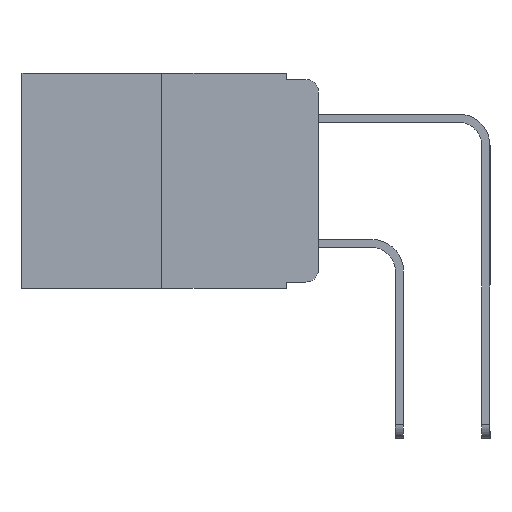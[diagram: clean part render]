
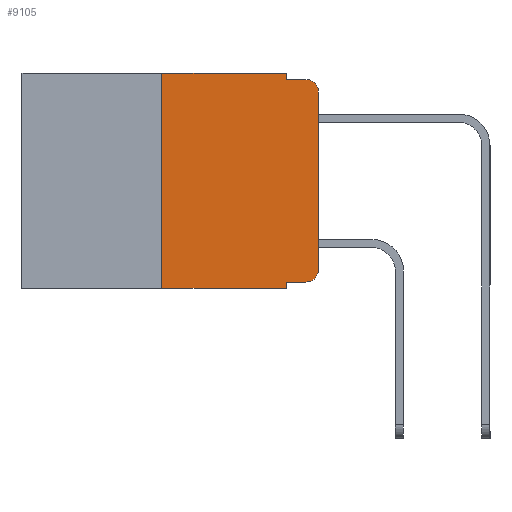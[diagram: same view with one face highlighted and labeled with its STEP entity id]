
A CAD part, left-side view. The second image highlights one B-rep face of the part: STEP entity #9105.
In plain terms, the highlighted planar face has unit normal (-1, 0, 0).
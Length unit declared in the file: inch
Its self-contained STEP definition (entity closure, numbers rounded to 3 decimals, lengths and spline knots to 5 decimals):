
#324 = EDGE_CURVE ( 'NONE', #7772, #11503, #10343, .T. ) ;
#444 = EDGE_LOOP ( 'NONE', ( #8422, #6084, #1787, #8151, #3072, #1596, #8136, #9040, #4002, #3532 ) ) ;
#584 = VECTOR ( 'NONE', #12914, 39.37008 ) ;
#625 = CARTESIAN_POINT ( 'NONE',  ( 0., 0.473, -0.343 ) ) ;
#909 = LINE ( 'NONE', #10225, #6600 ) ;
#931 = DIRECTION ( 'NONE',  ( 0., 0., 1. ) ) ;
#988 = AXIS2_PLACEMENT_3D ( 'NONE', #12004, #6109, #12974 ) ;
#1077 = LINE ( 'NONE', #11013, #2691 ) ;
#1115 = EDGE_CURVE ( 'NONE', #9015, #11503, #10169, .T. ) ;
#1596 = ORIENTED_EDGE ( 'NONE', *, *, #11687, .F. ) ;
#1787 = ORIENTED_EDGE ( 'NONE', *, *, #324, .F. ) ;
#1903 = CARTESIAN_POINT ( 'NONE',  ( 0., 0., -0.313 ) ) ;
#2172 = CIRCLE ( 'NONE', #988, 0.02 ) ;
#2373 = CARTESIAN_POINT ( 'NONE',  ( 0., 0.051, 0. ) ) ;
#2612 = VECTOR ( 'NONE', #7106, 39.37008 ) ;
#2691 = VECTOR ( 'NONE', #7093, 39.37008 ) ;
#3072 = ORIENTED_EDGE ( 'NONE', *, *, #8493, .F. ) ;
#3446 = CARTESIAN_POINT ( 'NONE',  ( 0., 0.02, -0.03 ) ) ;
#3532 = ORIENTED_EDGE ( 'NONE', *, *, #8409, .T. ) ;
#3619 = VERTEX_POINT ( 'NONE', #8544 ) ;
#3703 = VECTOR ( 'NONE', #10161, 39.37008 ) ;
#4002 = ORIENTED_EDGE ( 'NONE', *, *, #9057, .T. ) ;
#4096 = EDGE_CURVE ( 'NONE', #4557, #9015, #9463, .T. ) ;
#4107 = DIRECTION ( 'NONE',  ( 0., 0., 1. ) ) ;
#4124 = CARTESIAN_POINT ( 'NONE',  ( 0., 0., 0. ) ) ;
#4347 = LINE ( 'NONE', #7207, #3703 ) ;
#4447 = VECTOR ( 'NONE', #4107, 39.37008 ) ;
#4557 = VERTEX_POINT ( 'NONE', #1903 ) ;
#5051 = VECTOR ( 'NONE', #6520, 39.37008 ) ;
#5110 = CARTESIAN_POINT ( 'NONE',  ( 0., 0.473, 0. ) ) ;
#5154 = PLANE ( 'NONE',  #8866 ) ;
#5650 = EDGE_CURVE ( 'NONE', #7003, #11461, #6347, .T. ) ;
#5992 = CARTESIAN_POINT ( 'NONE',  ( 0., 0.051, -0.343 ) ) ;
#6007 = CARTESIAN_POINT ( 'NONE',  ( 0., 0., -0.03 ) ) ;
#6084 = ORIENTED_EDGE ( 'NONE', *, *, #1115, .T. ) ;
#6103 = CARTESIAN_POINT ( 'NONE',  ( 0., 0.051, 0. ) ) ;
#6109 = DIRECTION ( 'NONE',  ( -1., 0., 0. ) ) ;
#6126 = LINE ( 'NONE', #2373, #11063 ) ;
#6180 = DIRECTION ( 'NONE',  ( 1., 0., 0. ) ) ;
#6200 = VERTEX_POINT ( 'NONE', #7928 ) ;
#6218 = CARTESIAN_POINT ( 'NONE',  ( 0., 0.051, -0.01 ) ) ;
#6347 = LINE ( 'NONE', #625, #584 ) ;
#6520 = DIRECTION ( 'NONE',  ( 0., -1., 0. ) ) ;
#6600 = VECTOR ( 'NONE', #931, 39.37008 ) ;
#6816 = VERTEX_POINT ( 'NONE', #7728 ) ;
#6984 = CARTESIAN_POINT ( 'NONE',  ( 0., 0.051, -0.333 ) ) ;
#7003 = VERTEX_POINT ( 'NONE', #12969 ) ;
#7093 = DIRECTION ( 'NONE',  ( 0., -1., 0. ) ) ;
#7106 = DIRECTION ( 'NONE',  ( 0., 0., -1. ) ) ;
#7207 = CARTESIAN_POINT ( 'NONE',  ( 0., 0.473, 0. ) ) ;
#7341 = AXIS2_PLACEMENT_3D ( 'NONE', #3446, #13272, #13082 ) ;
#7681 = CARTESIAN_POINT ( 'NONE',  ( 0., 0.051, -0.01 ) ) ;
#7728 = CARTESIAN_POINT ( 'NONE',  ( 0., 0.25, 0. ) ) ;
#7772 = VERTEX_POINT ( 'NONE', #6218 ) ;
#7928 = CARTESIAN_POINT ( 'NONE',  ( 0., 0.051, 0. ) ) ;
#8136 = ORIENTED_EDGE ( 'NONE', *, *, #5650, .T. ) ;
#8151 = ORIENTED_EDGE ( 'NONE', *, *, #12329, .F. ) ;
#8262 = VERTEX_POINT ( 'NONE', #6984 ) ;
#8409 = EDGE_CURVE ( 'NONE', #3619, #4557, #2172, .T. ) ;
#8422 = ORIENTED_EDGE ( 'NONE', *, *, #4096, .T. ) ;
#8493 = EDGE_CURVE ( 'NONE', #6816, #6200, #4347, .T. ) ;
#8544 = CARTESIAN_POINT ( 'NONE',  ( 0., 0.02, -0.333 ) ) ;
#8866 = AXIS2_PLACEMENT_3D ( 'NONE', #5110, #6180, #13043 ) ;
#8977 = CARTESIAN_POINT ( 'NONE',  ( 0., 0.02, -0.01 ) ) ;
#9015 = VERTEX_POINT ( 'NONE', #6007 ) ;
#9040 = ORIENTED_EDGE ( 'NONE', *, *, #10370, .F. ) ;
#9057 = EDGE_CURVE ( 'NONE', #8262, #3619, #1077, .T. ) ;
#9105 = ADVANCED_FACE ( 'NONE', ( #12194 ), #5154, .F. ) ;
#9463 = LINE ( 'NONE', #4124, #4447 ) ;
#9497 = DIRECTION ( 'NONE',  ( 0., 0., -1. ) ) ;
#10161 = DIRECTION ( 'NONE',  ( 0., -1., 0. ) ) ;
#10169 = CIRCLE ( 'NONE', #7341, 0.02 ) ;
#10225 = CARTESIAN_POINT ( 'NONE',  ( 0., 0.25, 0. ) ) ;
#10343 = LINE ( 'NONE', #7681, #5051 ) ;
#10370 = EDGE_CURVE ( 'NONE', #8262, #11461, #13238, .T. ) ;
#11013 = CARTESIAN_POINT ( 'NONE',  ( 0., 0.051, -0.333 ) ) ;
#11063 = VECTOR ( 'NONE', #9497, 39.37008 ) ;
#11461 = VERTEX_POINT ( 'NONE', #5992 ) ;
#11503 = VERTEX_POINT ( 'NONE', #8977 ) ;
#11687 = EDGE_CURVE ( 'NONE', #7003, #6816, #909, .T. ) ;
#12004 = CARTESIAN_POINT ( 'NONE',  ( 0., 0.02, -0.313 ) ) ;
#12194 = FACE_OUTER_BOUND ( 'NONE', #444, .T. ) ;
#12329 = EDGE_CURVE ( 'NONE', #6200, #7772, #6126, .T. ) ;
#12914 = DIRECTION ( 'NONE',  ( 0., -1., 0. ) ) ;
#12969 = CARTESIAN_POINT ( 'NONE',  ( 0., 0.25, -0.343 ) ) ;
#12974 = DIRECTION ( 'NONE',  ( 0., 0., -1. ) ) ;
#13043 = DIRECTION ( 'NONE',  ( 0., 0., -1. ) ) ;
#13082 = DIRECTION ( 'NONE',  ( 0., 0., -1. ) ) ;
#13238 = LINE ( 'NONE', #6103, #2612 ) ;
#13272 = DIRECTION ( 'NONE',  ( -1., 0., 0. ) ) ;
